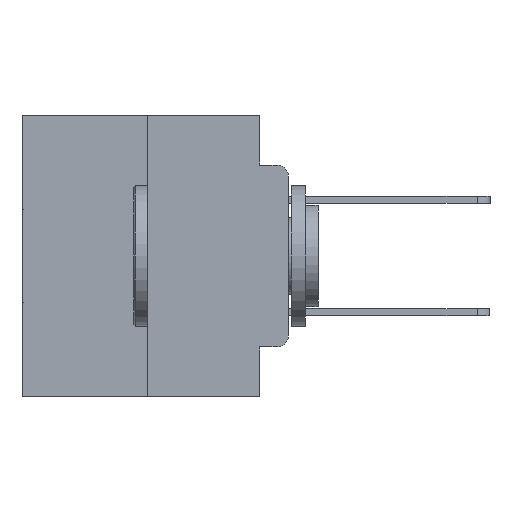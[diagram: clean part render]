
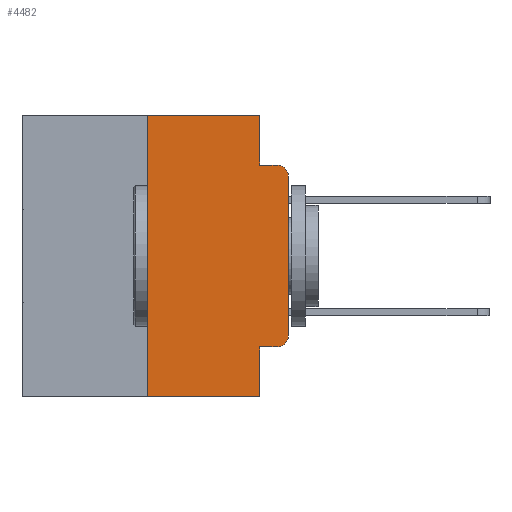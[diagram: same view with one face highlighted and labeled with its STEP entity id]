
A CAD part, left-side view. The second image highlights one B-rep face of the part: STEP entity #4482.
In plain terms, the highlighted planar face has unit normal (-1, 0, 0).
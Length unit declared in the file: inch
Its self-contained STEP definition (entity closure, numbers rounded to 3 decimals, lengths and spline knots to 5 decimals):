
#486 = DIRECTION ( 'NONE',  ( 0., 0., 1. ) ) ;
#866 = CARTESIAN_POINT ( 'NONE',  ( 0., 0.473, 0. ) ) ;
#1623 = EDGE_CURVE ( 'NONE', #2951, #16010, #26500, .T. ) ;
#1906 = ORIENTED_EDGE ( 'NONE', *, *, #12442, .T. ) ;
#1950 = DIRECTION ( 'NONE',  ( 1., 0., 0. ) ) ;
#1995 = VERTEX_POINT ( 'NONE', #27703 ) ;
#2367 = CARTESIAN_POINT ( 'NONE',  ( 0., 0.051, 0. ) ) ;
#2483 = VECTOR ( 'NONE', #27745, 39.37008 ) ;
#2951 = VERTEX_POINT ( 'NONE', #16897 ) ;
#4482 = ADVANCED_FACE ( 'NONE', ( #25615 ), #30367, .F. ) ;
#5492 = ORIENTED_EDGE ( 'NONE', *, *, #13797, .F. ) ;
#5862 = ORIENTED_EDGE ( 'NONE', *, *, #27949, .F. ) ;
#5876 = VERTEX_POINT ( 'NONE', #18783 ) ;
#6623 = AXIS2_PLACEMENT_3D ( 'NONE', #16210, #1950, #18658 ) ;
#6643 = DIRECTION ( 'NONE',  ( 0., 0., -1. ) ) ;
#6861 = VECTOR ( 'NONE', #25042, 39.37008 ) ;
#7002 = LINE ( 'NONE', #28953, #12588 ) ;
#7423 = LINE ( 'NONE', #11613, #20079 ) ;
#7699 = EDGE_CURVE ( 'NONE', #21585, #30619, #19784, .T. ) ;
#7709 = VERTEX_POINT ( 'NONE', #12916 ) ;
#8109 = LINE ( 'NONE', #11639, #19992 ) ;
#8161 = CARTESIAN_POINT ( 'NONE',  ( 0., 0.051, -0.5 ) ) ;
#8446 = DIRECTION ( 'NONE',  ( 0., -1., 0. ) ) ;
#8679 = CARTESIAN_POINT ( 'NONE',  ( 0., 0., -0.1085 ) ) ;
#9000 = ORIENTED_EDGE ( 'NONE', *, *, #30420, .T. ) ;
#9035 = CIRCLE ( 'NONE', #14402, 0.02 ) ;
#10529 = DIRECTION ( 'NONE',  ( 0., -1., 0. ) ) ;
#11060 = VECTOR ( 'NONE', #6643, 39.37008 ) ;
#11613 = CARTESIAN_POINT ( 'NONE',  ( 0., 0.25, 0. ) ) ;
#11639 = CARTESIAN_POINT ( 'NONE',  ( 0., 0.051, 0. ) ) ;
#12314 = CARTESIAN_POINT ( 'NONE',  ( 0., 0.02, -0.1085 ) ) ;
#12442 = EDGE_CURVE ( 'NONE', #7709, #12696, #9035, .T. ) ;
#12588 = VECTOR ( 'NONE', #486, 39.37008 ) ;
#12696 = VERTEX_POINT ( 'NONE', #14348 ) ;
#12916 = CARTESIAN_POINT ( 'NONE',  ( 0., 0.02, -0.4115 ) ) ;
#13467 = VECTOR ( 'NONE', #10529, 39.37008 ) ;
#13555 = DIRECTION ( 'NONE',  ( -1., 0., 0. ) ) ;
#13709 = CARTESIAN_POINT ( 'NONE',  ( 0., 0.051, 0. ) ) ;
#13797 = EDGE_CURVE ( 'NONE', #2951, #21585, #7423, .T. ) ;
#14115 = ORIENTED_EDGE ( 'NONE', *, *, #1623, .T. ) ;
#14348 = CARTESIAN_POINT ( 'NONE',  ( 0., 0., -0.3915 ) ) ;
#14402 = AXIS2_PLACEMENT_3D ( 'NONE', #27724, #13555, #30057 ) ;
#14671 = DIRECTION ( 'NONE',  ( 0., 0., -1. ) ) ;
#15125 = EDGE_CURVE ( 'NONE', #5876, #16010, #8109, .T. ) ;
#16010 = VERTEX_POINT ( 'NONE', #8161 ) ;
#16120 = VERTEX_POINT ( 'NONE', #8679 ) ;
#16210 = CARTESIAN_POINT ( 'NONE',  ( 0., 0.473, 0. ) ) ;
#16310 = VECTOR ( 'NONE', #8446, 39.37008 ) ;
#16523 = VERTEX_POINT ( 'NONE', #30446 ) ;
#16647 = ORIENTED_EDGE ( 'NONE', *, *, #7699, .F. ) ;
#16897 = CARTESIAN_POINT ( 'NONE',  ( 0., 0.25, -0.5 ) ) ;
#17310 = LINE ( 'NONE', #13709, #11060 ) ;
#17831 = LINE ( 'NONE', #27365, #16310 ) ;
#18658 = DIRECTION ( 'NONE',  ( 0., 0., -1. ) ) ;
#18683 = DIRECTION ( 'NONE',  ( 0., 0., -1. ) ) ;
#18783 = CARTESIAN_POINT ( 'NONE',  ( 0., 0.051, -0.4115 ) ) ;
#18902 = ORIENTED_EDGE ( 'NONE', *, *, #28931, .T. ) ;
#19784 = LINE ( 'NONE', #866, #13467 ) ;
#19992 = VECTOR ( 'NONE', #18683, 39.37008 ) ;
#20079 = VECTOR ( 'NONE', #28140, 39.37008 ) ;
#20468 = ORIENTED_EDGE ( 'NONE', *, *, #15125, .F. ) ;
#20749 = CARTESIAN_POINT ( 'NONE',  ( 0., 0.051, -0.4115 ) ) ;
#21290 = EDGE_LOOP ( 'NONE', ( #29565, #18902, #28856, #5862, #16647, #5492, #14115, #20468, #9000, #1906 ) ) ;
#21569 = CARTESIAN_POINT ( 'NONE',  ( 0., 0.473, -0.5 ) ) ;
#21585 = VERTEX_POINT ( 'NONE', #30506 ) ;
#23634 = AXIS2_PLACEMENT_3D ( 'NONE', #12314, #28842, #14671 ) ;
#25042 = DIRECTION ( 'NONE',  ( 0., -1., 0. ) ) ;
#25615 = FACE_OUTER_BOUND ( 'NONE', #21290, .T. ) ;
#25975 = EDGE_CURVE ( 'NONE', #1995, #16523, #17831, .T. ) ;
#26500 = LINE ( 'NONE', #21569, #6861 ) ;
#27365 = CARTESIAN_POINT ( 'NONE',  ( 0., 0.051, -0.0885 ) ) ;
#27703 = CARTESIAN_POINT ( 'NONE',  ( 0., 0.051, -0.0885 ) ) ;
#27724 = CARTESIAN_POINT ( 'NONE',  ( 0., 0.02, -0.3915 ) ) ;
#27745 = DIRECTION ( 'NONE',  ( 0., -1., 0. ) ) ;
#27771 = LINE ( 'NONE', #20749, #2483 ) ;
#27949 = EDGE_CURVE ( 'NONE', #30619, #1995, #17310, .T. ) ;
#28140 = DIRECTION ( 'NONE',  ( 0., 0., 1. ) ) ;
#28360 = CIRCLE ( 'NONE', #23634, 0.02 ) ;
#28842 = DIRECTION ( 'NONE',  ( -1., 0., 0. ) ) ;
#28856 = ORIENTED_EDGE ( 'NONE', *, *, #25975, .F. ) ;
#28931 = EDGE_CURVE ( 'NONE', #16120, #16523, #28360, .T. ) ;
#28953 = CARTESIAN_POINT ( 'NONE',  ( 0., 0., 0. ) ) ;
#29565 = ORIENTED_EDGE ( 'NONE', *, *, #30724, .T. ) ;
#30057 = DIRECTION ( 'NONE',  ( 0., 0., -1. ) ) ;
#30367 = PLANE ( 'NONE',  #6623 ) ;
#30420 = EDGE_CURVE ( 'NONE', #5876, #7709, #27771, .T. ) ;
#30446 = CARTESIAN_POINT ( 'NONE',  ( 0., 0.02, -0.0885 ) ) ;
#30506 = CARTESIAN_POINT ( 'NONE',  ( 0., 0.25, 0. ) ) ;
#30619 = VERTEX_POINT ( 'NONE', #2367 ) ;
#30724 = EDGE_CURVE ( 'NONE', #12696, #16120, #7002, .T. ) ;
